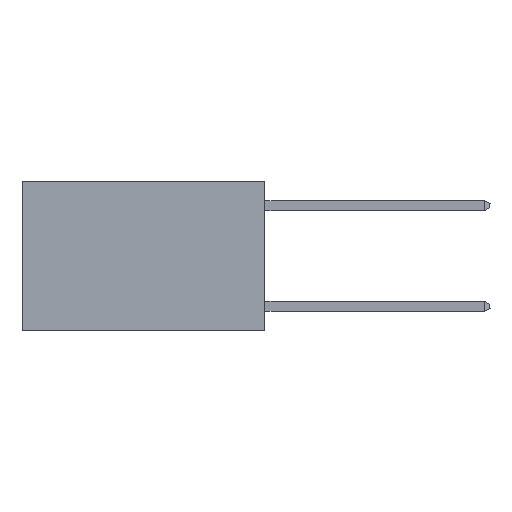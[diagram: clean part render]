
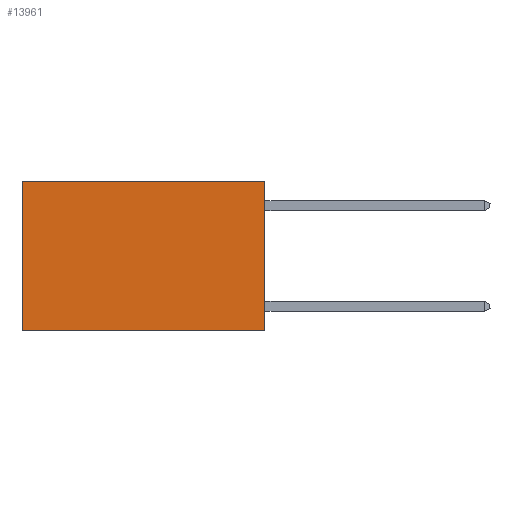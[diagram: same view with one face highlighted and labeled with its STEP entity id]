
A CAD part, left-side view. The second image highlights one B-rep face of the part: STEP entity #13961.
In plain terms, the highlighted planar face has unit normal (-1, 0, 0).
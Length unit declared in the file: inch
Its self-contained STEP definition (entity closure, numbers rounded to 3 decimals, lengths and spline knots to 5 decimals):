
#44 = CARTESIAN_POINT ( 'NONE',  ( 0.2625, 0., -0.37 ) ) ;
#95 = EDGE_CURVE ( 'NONE', #14224, #5627, #1655, .T. ) ;
#543 = VECTOR ( 'NONE', #12842, 39.37008 ) ;
#1574 = ORIENTED_EDGE ( 'NONE', *, *, #95, .F. ) ;
#1655 = LINE ( 'NONE', #5379, #3899 ) ;
#1832 = VECTOR ( 'NONE', #11273, 39.37008 ) ;
#2491 = FACE_OUTER_BOUND ( 'NONE', #14543, .T. ) ;
#2505 = LINE ( 'NONE', #14094, #543 ) ;
#3899 = VECTOR ( 'NONE', #11156, 39.37008 ) ;
#4138 = CARTESIAN_POINT ( 'NONE',  ( 0.2625, 0., 0. ) ) ;
#4181 = VERTEX_POINT ( 'NONE', #10548 ) ;
#5172 = LINE ( 'NONE', #6474, #13372 ) ;
#5379 = CARTESIAN_POINT ( 'NONE',  ( 0.2625, 0., 0. ) ) ;
#5627 = VERTEX_POINT ( 'NONE', #44 ) ;
#6474 = CARTESIAN_POINT ( 'NONE',  ( 0.2625, 0., -0.37 ) ) ;
#6752 = EDGE_CURVE ( 'NONE', #14224, #4181, #11121, .T. ) ;
#6920 = PLANE ( 'NONE',  #7764 ) ;
#7404 = DIRECTION ( 'NONE',  ( 0., 1., 0. ) ) ;
#7618 = ORIENTED_EDGE ( 'NONE', *, *, #6752, .T. ) ;
#7764 = AXIS2_PLACEMENT_3D ( 'NONE', #15166, #14151, #13923 ) ;
#8972 = CARTESIAN_POINT ( 'NONE',  ( 0.2625, 0., 0. ) ) ;
#10405 = CARTESIAN_POINT ( 'NONE',  ( 0.2625, 0.6, -0.37 ) ) ;
#10548 = CARTESIAN_POINT ( 'NONE',  ( 0.2625, 0.6, 0. ) ) ;
#11087 = ORIENTED_EDGE ( 'NONE', *, *, #11845, .F. ) ;
#11121 = LINE ( 'NONE', #8972, #1832 ) ;
#11156 = DIRECTION ( 'NONE',  ( 0., 0., -1. ) ) ;
#11273 = DIRECTION ( 'NONE',  ( 0., 1., 0. ) ) ;
#11308 = EDGE_CURVE ( 'NONE', #4181, #12212, #2505, .T. ) ;
#11845 = EDGE_CURVE ( 'NONE', #5627, #12212, #5172, .T. ) ;
#12212 = VERTEX_POINT ( 'NONE', #10405 ) ;
#12523 = ORIENTED_EDGE ( 'NONE', *, *, #11308, .T. ) ;
#12842 = DIRECTION ( 'NONE',  ( 0., 0., -1. ) ) ;
#13372 = VECTOR ( 'NONE', #7404, 39.37008 ) ;
#13923 = DIRECTION ( 'NONE',  ( 0., 0., -1. ) ) ;
#13961 = ADVANCED_FACE ( 'NONE', ( #2491 ), #6920, .F. ) ;
#14094 = CARTESIAN_POINT ( 'NONE',  ( 0.2625, 0.6, 0. ) ) ;
#14151 = DIRECTION ( 'NONE',  ( 1., 0., 0. ) ) ;
#14224 = VERTEX_POINT ( 'NONE', #4138 ) ;
#14543 = EDGE_LOOP ( 'NONE', ( #12523, #11087, #1574, #7618 ) ) ;
#15166 = CARTESIAN_POINT ( 'NONE',  ( 0.2625, 0., 0. ) ) ;
